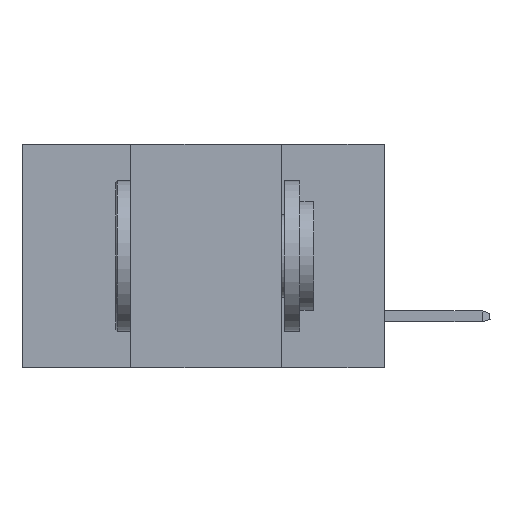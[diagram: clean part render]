
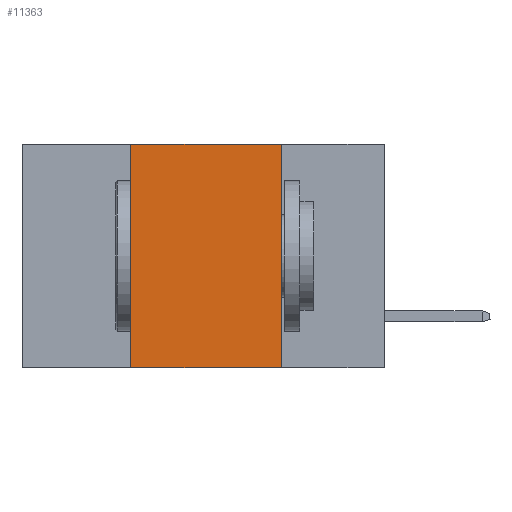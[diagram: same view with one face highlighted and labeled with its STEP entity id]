
A CAD part, left-side view. The second image highlights one B-rep face of the part: STEP entity #11363.
In plain terms, the highlighted planar face has unit normal (-1, 0, 0).
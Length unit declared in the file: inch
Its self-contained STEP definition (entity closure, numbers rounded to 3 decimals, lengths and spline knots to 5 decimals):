
#46 = VERTEX_POINT ( 'NONE', #2867 ) ;
#318 = LINE ( 'NONE', #13960, #8765 ) ;
#564 = FACE_OUTER_BOUND ( 'NONE', #5497, .T. ) ;
#1374 = VERTEX_POINT ( 'NONE', #8469 ) ;
#2317 = CARTESIAN_POINT ( 'NONE',  ( 0., 0.6, 0. ) ) ;
#2337 = CARTESIAN_POINT ( 'NONE',  ( 0., 0.17, 0. ) ) ;
#2760 = VECTOR ( 'NONE', #6176, 39.37008 ) ;
#2867 = CARTESIAN_POINT ( 'NONE',  ( 0., 0.17, -0.37 ) ) ;
#3411 = CARTESIAN_POINT ( 'NONE',  ( 0., 0.42, -0.37 ) ) ;
#4519 = PLANE ( 'NONE',  #14887 ) ;
#4680 = ORIENTED_EDGE ( 'NONE', *, *, #8373, .T. ) ;
#4760 = DIRECTION ( 'NONE',  ( 0., -1., 0. ) ) ;
#4851 = EDGE_CURVE ( 'NONE', #8790, #46, #12436, .T. ) ;
#4944 = DIRECTION ( 'NONE',  ( 0., -1., 0. ) ) ;
#5169 = EDGE_CURVE ( 'NONE', #1374, #8790, #10656, .T. ) ;
#5497 = EDGE_LOOP ( 'NONE', ( #13228, #14581, #14699, #4680 ) ) ;
#6176 = DIRECTION ( 'NONE',  ( 0., 0., 1. ) ) ;
#7084 = LINE ( 'NONE', #12112, #2760 ) ;
#7585 = VECTOR ( 'NONE', #4760, 39.37008 ) ;
#8373 = EDGE_CURVE ( 'NONE', #8605, #46, #318, .T. ) ;
#8469 = CARTESIAN_POINT ( 'NONE',  ( 0., 0.42, 0. ) ) ;
#8605 = VERTEX_POINT ( 'NONE', #3411 ) ;
#8765 = VECTOR ( 'NONE', #4944, 39.37008 ) ;
#8790 = VERTEX_POINT ( 'NONE', #2337 ) ;
#9394 = VECTOR ( 'NONE', #12356, 39.37008 ) ;
#10229 = EDGE_CURVE ( 'NONE', #8605, #1374, #7084, .T. ) ;
#10656 = LINE ( 'NONE', #2317, #7585 ) ;
#11363 = ADVANCED_FACE ( 'NONE', ( #564 ), #4519, .F. ) ;
#11693 = DIRECTION ( 'NONE',  ( 1., 0., 0. ) ) ;
#11996 = CARTESIAN_POINT ( 'NONE',  ( 0., 0.17, 0. ) ) ;
#12112 = CARTESIAN_POINT ( 'NONE',  ( 0., 0.42, 0. ) ) ;
#12356 = DIRECTION ( 'NONE',  ( 0., 0., -1. ) ) ;
#12436 = LINE ( 'NONE', #11996, #9394 ) ;
#12540 = CARTESIAN_POINT ( 'NONE',  ( 0., 0.6, 0. ) ) ;
#12890 = DIRECTION ( 'NONE',  ( 0., 0., -1. ) ) ;
#13228 = ORIENTED_EDGE ( 'NONE', *, *, #4851, .F. ) ;
#13960 = CARTESIAN_POINT ( 'NONE',  ( 0., 0.6, -0.37 ) ) ;
#14581 = ORIENTED_EDGE ( 'NONE', *, *, #5169, .F. ) ;
#14699 = ORIENTED_EDGE ( 'NONE', *, *, #10229, .F. ) ;
#14887 = AXIS2_PLACEMENT_3D ( 'NONE', #12540, #11693, #12890 ) ;
